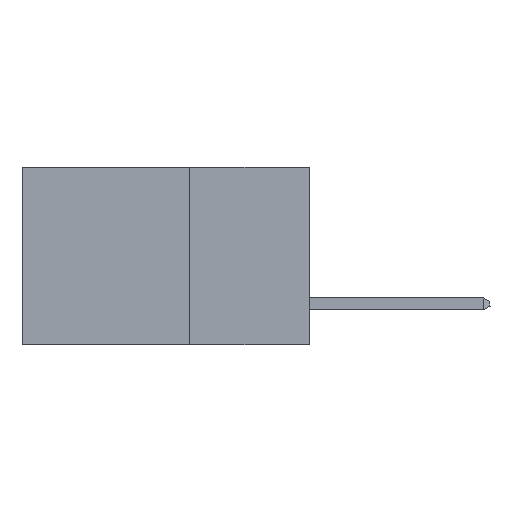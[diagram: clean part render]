
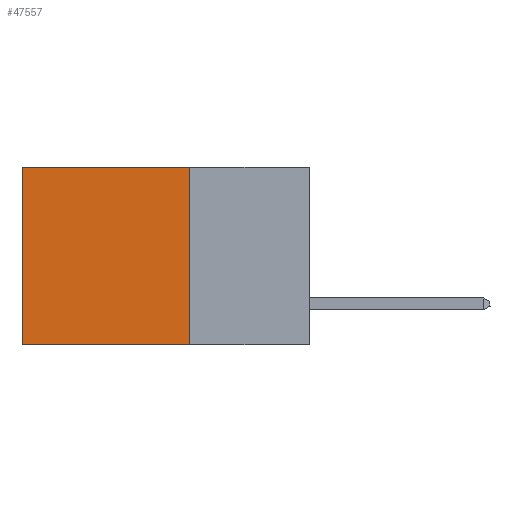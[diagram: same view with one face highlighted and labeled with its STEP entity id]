
A CAD part, left-side view. The second image highlights one B-rep face of the part: STEP entity #47557.
In plain terms, the highlighted planar face has unit normal (-1, 0, 0).
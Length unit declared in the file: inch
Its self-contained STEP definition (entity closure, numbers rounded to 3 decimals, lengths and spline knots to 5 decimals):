
#30 = ORIENTED_EDGE ( 'NONE', *, *, #21884, .F. ) ;
#1693 = CARTESIAN_POINT ( 'NONE',  ( 0.2875, 0.25, -0.37 ) ) ;
#2168 = CARTESIAN_POINT ( 'NONE',  ( 0.2875, 0.6, 0. ) ) ;
#4713 = DIRECTION ( 'NONE',  ( 0., 1., 0. ) ) ;
#6208 = CARTESIAN_POINT ( 'NONE',  ( 0.2875, 0.25, -0.37 ) ) ;
#6289 = DIRECTION ( 'NONE',  ( 0., 0., -1. ) ) ;
#7902 = VERTEX_POINT ( 'NONE', #38895 ) ;
#9119 = CARTESIAN_POINT ( 'NONE',  ( 0.2875, 0.25, 0. ) ) ;
#10037 = CARTESIAN_POINT ( 'NONE',  ( 0.2875, 0.6, 0. ) ) ;
#11551 = ORIENTED_EDGE ( 'NONE', *, *, #48816, .T. ) ;
#13224 = FACE_OUTER_BOUND ( 'NONE', #26068, .T. ) ;
#14348 = LINE ( 'NONE', #1693, #37323 ) ;
#17078 = LINE ( 'NONE', #9119, #35973 ) ;
#18560 = EDGE_CURVE ( 'NONE', #44238, #32907, #14348, .T. ) ;
#20776 = VECTOR ( 'NONE', #6289, 39.37008 ) ;
#21224 = DIRECTION ( 'NONE',  ( 0., 0., -1. ) ) ;
#21884 = EDGE_CURVE ( 'NONE', #7902, #44238, #25981, .T. ) ;
#24208 = VECTOR ( 'NONE', #21224, 39.37008 ) ;
#24374 = ORIENTED_EDGE ( 'NONE', *, *, #46035, .T. ) ;
#24815 = PLANE ( 'NONE',  #30489 ) ;
#25020 = CARTESIAN_POINT ( 'NONE',  ( 0.2875, 0.25, 0. ) ) ;
#25981 = LINE ( 'NONE', #25020, #24208 ) ;
#26068 = EDGE_LOOP ( 'NONE', ( #11551, #39333, #30, #24374 ) ) ;
#27242 = LINE ( 'NONE', #2168, #20776 ) ;
#30489 = AXIS2_PLACEMENT_3D ( 'NONE', #40027, #47959, #43989 ) ;
#31717 = CARTESIAN_POINT ( 'NONE',  ( 0.2875, 0.6, -0.37 ) ) ;
#31810 = DIRECTION ( 'NONE',  ( 0., 1., 0. ) ) ;
#32907 = VERTEX_POINT ( 'NONE', #31717 ) ;
#35973 = VECTOR ( 'NONE', #4713, 39.37008 ) ;
#37323 = VECTOR ( 'NONE', #31810, 39.37008 ) ;
#38895 = CARTESIAN_POINT ( 'NONE',  ( 0.2875, 0.25, 0. ) ) ;
#39333 = ORIENTED_EDGE ( 'NONE', *, *, #18560, .F. ) ;
#40027 = CARTESIAN_POINT ( 'NONE',  ( 0.2875, 0.25, 0. ) ) ;
#43989 = DIRECTION ( 'NONE',  ( 0., 0., -1. ) ) ;
#44238 = VERTEX_POINT ( 'NONE', #6208 ) ;
#45191 = VERTEX_POINT ( 'NONE', #10037 ) ;
#46035 = EDGE_CURVE ( 'NONE', #7902, #45191, #17078, .T. ) ;
#47557 = ADVANCED_FACE ( 'NONE', ( #13224 ), #24815, .F. ) ;
#47959 = DIRECTION ( 'NONE',  ( 1., 0., 0. ) ) ;
#48816 = EDGE_CURVE ( 'NONE', #45191, #32907, #27242, .T. ) ;
